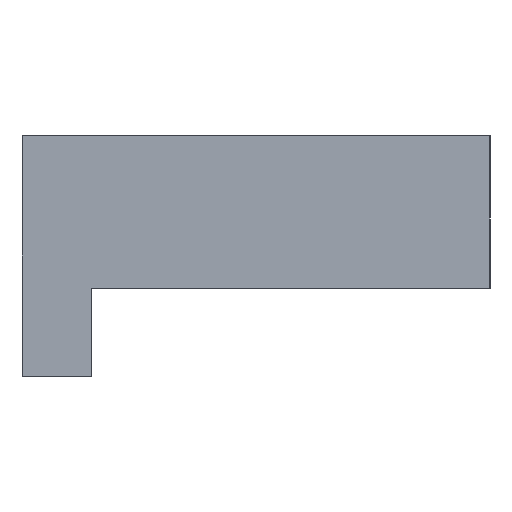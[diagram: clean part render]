
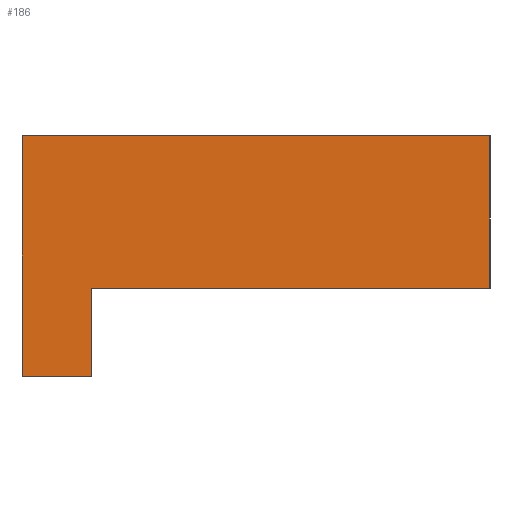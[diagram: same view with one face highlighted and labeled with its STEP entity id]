
A CAD part, left-side view. The second image highlights one B-rep face of the part: STEP entity #186.
In plain terms, the highlighted planar face has unit normal (-1, 0, 0).
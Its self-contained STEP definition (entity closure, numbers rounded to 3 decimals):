
#18=LINE('',#290,#36);
#19=LINE('',#293,#37);
#24=LINE('',#304,#42);
#27=LINE('',#308,#45);
#30=LINE('',#315,#48);
#31=LINE('',#316,#49);
#36=VECTOR('',#242,10.);
#37=VECTOR('',#245,10.);
#42=VECTOR('',#252,10.);
#45=VECTOR('',#257,10.);
#48=VECTOR('',#264,10.);
#49=VECTOR('',#265,10.);
#56=PLANE('',#220);
#72=FACE_OUTER_BOUND('',#86,.T.);
#86=EDGE_LOOP('',(#161,#162,#163,#164,#165,#166));
#99=VERTEX_POINT('',#283);
#102=VERTEX_POINT('',#288);
#103=VERTEX_POINT('',#292);
#107=VERTEX_POINT('',#301);
#108=VERTEX_POINT('',#303);
#110=VERTEX_POINT('',#314);
#118=EDGE_CURVE('',#99,#102,#18,.T.);
#119=EDGE_CURVE('',#99,#103,#19,.T.);
#124=EDGE_CURVE('',#108,#107,#24,.T.);
#127=EDGE_CURVE('',#103,#107,#27,.T.);
#130=EDGE_CURVE('',#110,#102,#30,.T.);
#131=EDGE_CURVE('',#108,#110,#31,.T.);
#161=ORIENTED_EDGE('',*,*,#124,.T.);
#162=ORIENTED_EDGE('',*,*,#127,.F.);
#163=ORIENTED_EDGE('',*,*,#119,.F.);
#164=ORIENTED_EDGE('',*,*,#118,.T.);
#165=ORIENTED_EDGE('',*,*,#130,.F.);
#166=ORIENTED_EDGE('',*,*,#131,.F.);
#186=ADVANCED_FACE('',(#72),#56,.F.);
#220=AXIS2_PLACEMENT_3D('',#313,#262,#263);
#242=DIRECTION('',(0.,-1.,0.));
#245=DIRECTION('',(0.,0.,-1.));
#252=DIRECTION('',(0.,0.,-1.));
#257=DIRECTION('',(0.,1.,0.));
#262=DIRECTION('center_axis',(1.,0.,0.));
#263=DIRECTION('ref_axis',(0.,-1.,0.));
#264=DIRECTION('',(0.,0.,-1.));
#265=DIRECTION('',(0.,-1.,0.));
#283=CARTESIAN_POINT('',(2.134,0.84,-10.036));
#288=CARTESIAN_POINT('',(2.134,-5.782,-10.036));
#290=CARTESIAN_POINT('',(2.134,1.92,-10.036));
#292=CARTESIAN_POINT('',(2.134,0.84,-11.5));
#293=CARTESIAN_POINT('',(2.134,0.84,-9.5));
#301=CARTESIAN_POINT('',(2.134,2.,-11.5));
#303=CARTESIAN_POINT('',(2.134,2.,-7.5));
#304=CARTESIAN_POINT('',(2.134,2.,-7.5));
#308=CARTESIAN_POINT('',(2.134,-6.875,-11.5));
#313=CARTESIAN_POINT('Origin',(2.134,2.5,-7.5));
#314=CARTESIAN_POINT('',(2.134,-5.782,-7.5));
#315=CARTESIAN_POINT('',(2.134,-5.782,-7.5));
#316=CARTESIAN_POINT('',(2.134,-6.875,-7.5));
